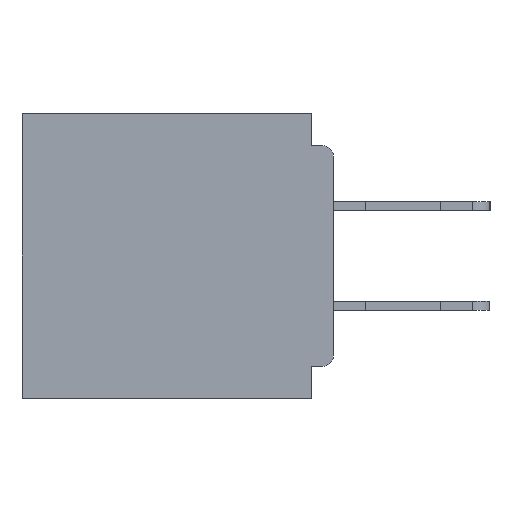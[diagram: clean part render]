
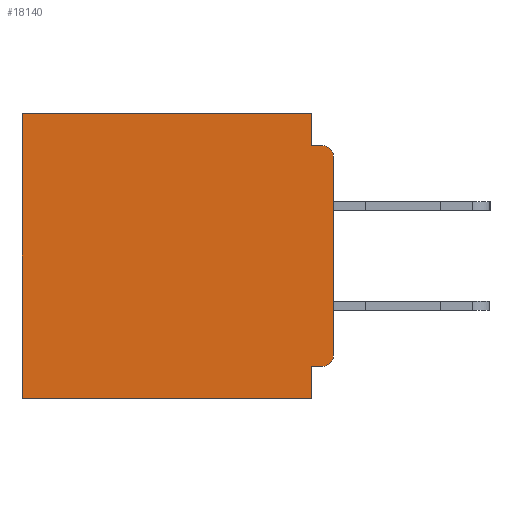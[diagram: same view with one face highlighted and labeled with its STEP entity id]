
A CAD part, left-side view. The second image highlights one B-rep face of the part: STEP entity #18140.
In plain terms, the highlighted planar face has unit normal (-1, 0, 0).
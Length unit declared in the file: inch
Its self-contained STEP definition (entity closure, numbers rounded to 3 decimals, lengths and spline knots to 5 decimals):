
#1460 = FACE_OUTER_BOUND ( 'NONE', #38488, .T. ) ;
#1604 = DIRECTION ( 'NONE',  ( 0., 0., -1. ) ) ;
#1790 = EDGE_CURVE ( 'NONE', #33776, #21565, #19119, .T. ) ;
#1946 = CARTESIAN_POINT ( 'NONE',  ( 0.3, 0., -0.4 ) ) ;
#2280 = LINE ( 'NONE', #10633, #11112 ) ;
#2460 = EDGE_CURVE ( 'NONE', #18944, #6877, #17499, .T. ) ;
#2597 = EDGE_CURVE ( 'NONE', #33776, #18944, #38839, .T. ) ;
#2975 = LINE ( 'NONE', #30619, #36220 ) ;
#3248 = CARTESIAN_POINT ( 'NONE',  ( 0.3, 0.015, -0.06 ) ) ;
#3604 = LINE ( 'NONE', #35738, #29031 ) ;
#5275 = VERTEX_POINT ( 'NONE', #12614 ) ;
#5469 = EDGE_CURVE ( 'NONE', #5275, #33750, #2280, .T. ) ;
#6628 = DIRECTION ( 'NONE',  ( 0., 0., -1. ) ) ;
#6877 = VERTEX_POINT ( 'NONE', #37821 ) ;
#7476 = DIRECTION ( 'NONE',  ( 0., 0., -1. ) ) ;
#7582 = PLANE ( 'NONE',  #20392 ) ;
#7740 = AXIS2_PLACEMENT_3D ( 'NONE', #25195, #25282, #26534 ) ;
#8827 = CARTESIAN_POINT ( 'NONE',  ( 0.3, 0.031, -0.355 ) ) ;
#10633 = CARTESIAN_POINT ( 'NONE',  ( 0.3, 0.437, -0.4 ) ) ;
#10864 = DIRECTION ( 'NONE',  ( 0., 0., -1. ) ) ;
#11112 = VECTOR ( 'NONE', #1604, 39.37008 ) ;
#12614 = CARTESIAN_POINT ( 'NONE',  ( 0.3, 0.437, 0. ) ) ;
#14399 = LINE ( 'NONE', #31849, #31014 ) ;
#14525 = CARTESIAN_POINT ( 'NONE',  ( 0.3, 0.031, 0. ) ) ;
#14537 = VERTEX_POINT ( 'NONE', #35769 ) ;
#16819 = ORIENTED_EDGE ( 'NONE', *, *, #2597, .F. ) ;
#17352 = VERTEX_POINT ( 'NONE', #14525 ) ;
#17499 = LINE ( 'NONE', #31809, #36252 ) ;
#17772 = LINE ( 'NONE', #1946, #41174 ) ;
#18140 = ADVANCED_FACE ( 'NONE', ( #1460 ), #7582, .F. ) ;
#18143 = VECTOR ( 'NONE', #19494, 39.37008 ) ;
#18463 = EDGE_CURVE ( 'NONE', #38807, #14537, #14399, .T. ) ;
#18944 = VERTEX_POINT ( 'NONE', #8827 ) ;
#18976 = CARTESIAN_POINT ( 'NONE',  ( 0.3, 0.031, -0.045 ) ) ;
#19119 = CIRCLE ( 'NONE', #7740, 0.015 ) ;
#19195 = LINE ( 'NONE', #42731, #18143 ) ;
#19494 = DIRECTION ( 'NONE',  ( 0., 1., 0. ) ) ;
#20392 = AXIS2_PLACEMENT_3D ( 'NONE', #20689, #30729, #10864 ) ;
#20689 = CARTESIAN_POINT ( 'NONE',  ( 0.3, 0., -0.4 ) ) ;
#20958 = CARTESIAN_POINT ( 'NONE',  ( 0.3, 0., -0.06 ) ) ;
#20993 = ORIENTED_EDGE ( 'NONE', *, *, #29904, .F. ) ;
#21375 = DIRECTION ( 'NONE',  ( 0., 1., 0. ) ) ;
#21565 = VERTEX_POINT ( 'NONE', #23058 ) ;
#21890 = CARTESIAN_POINT ( 'NONE',  ( 0.3, 0.015, -0.355 ) ) ;
#22543 = ORIENTED_EDGE ( 'NONE', *, *, #1790, .T. ) ;
#22721 = DIRECTION ( 'NONE',  ( 0., 0., -1. ) ) ;
#23058 = CARTESIAN_POINT ( 'NONE',  ( 0.3, 0., -0.34 ) ) ;
#23232 = EDGE_CURVE ( 'NONE', #17352, #5275, #3604, .T. ) ;
#23629 = ORIENTED_EDGE ( 'NONE', *, *, #33140, .F. ) ;
#24172 = AXIS2_PLACEMENT_3D ( 'NONE', #3248, #26444, #6628 ) ;
#25156 = ORIENTED_EDGE ( 'NONE', *, *, #18463, .F. ) ;
#25195 = CARTESIAN_POINT ( 'NONE',  ( 0.3, 0.015, -0.34 ) ) ;
#25282 = DIRECTION ( 'NONE',  ( -1., 0., 0. ) ) ;
#25742 = ORIENTED_EDGE ( 'NONE', *, *, #34652, .F. ) ;
#25830 = DIRECTION ( 'NONE',  ( 0., 1., 0. ) ) ;
#26357 = CIRCLE ( 'NONE', #24172, 0.015 ) ;
#26444 = DIRECTION ( 'NONE',  ( -1., 0., 0. ) ) ;
#26534 = DIRECTION ( 'NONE',  ( 0., 0., -1. ) ) ;
#27410 = VERTEX_POINT ( 'NONE', #20958 ) ;
#27508 = CARTESIAN_POINT ( 'NONE',  ( 0.3, 0., -0.355 ) ) ;
#28275 = CARTESIAN_POINT ( 'NONE',  ( 0.3, 0.437, -0.4 ) ) ;
#28468 = DIRECTION ( 'NONE',  ( 0., 0., -1. ) ) ;
#28781 = ORIENTED_EDGE ( 'NONE', *, *, #2460, .F. ) ;
#29031 = VECTOR ( 'NONE', #25830, 39.37008 ) ;
#29904 = EDGE_CURVE ( 'NONE', #17352, #38807, #2975, .T. ) ;
#29963 = VECTOR ( 'NONE', #21375, 39.37008 ) ;
#30619 = CARTESIAN_POINT ( 'NONE',  ( 0.3, 0.031, 0. ) ) ;
#30729 = DIRECTION ( 'NONE',  ( 1., 0., 0. ) ) ;
#31014 = VECTOR ( 'NONE', #42750, 39.37008 ) ;
#31444 = ORIENTED_EDGE ( 'NONE', *, *, #5469, .T. ) ;
#31809 = CARTESIAN_POINT ( 'NONE',  ( 0.3, 0.031, -0.4 ) ) ;
#31849 = CARTESIAN_POINT ( 'NONE',  ( 0.3, 0., -0.045 ) ) ;
#33140 = EDGE_CURVE ( 'NONE', #27410, #21565, #17772, .T. ) ;
#33750 = VERTEX_POINT ( 'NONE', #28275 ) ;
#33776 = VERTEX_POINT ( 'NONE', #21890 ) ;
#34652 = EDGE_CURVE ( 'NONE', #6877, #33750, #19195, .T. ) ;
#35738 = CARTESIAN_POINT ( 'NONE',  ( 0.3, 0., 0. ) ) ;
#35769 = CARTESIAN_POINT ( 'NONE',  ( 0.3, 0.015, -0.045 ) ) ;
#36220 = VECTOR ( 'NONE', #7476, 39.37008 ) ;
#36252 = VECTOR ( 'NONE', #22721, 39.37008 ) ;
#37821 = CARTESIAN_POINT ( 'NONE',  ( 0.3, 0.031, -0.4 ) ) ;
#38334 = EDGE_CURVE ( 'NONE', #27410, #14537, #26357, .T. ) ;
#38488 = EDGE_LOOP ( 'NONE', ( #23629, #40273, #25156, #20993, #40834, #31444, #25742, #28781, #16819, #22543 ) ) ;
#38807 = VERTEX_POINT ( 'NONE', #18976 ) ;
#38839 = LINE ( 'NONE', #27508, #29963 ) ;
#40273 = ORIENTED_EDGE ( 'NONE', *, *, #38334, .T. ) ;
#40834 = ORIENTED_EDGE ( 'NONE', *, *, #23232, .T. ) ;
#41174 = VECTOR ( 'NONE', #28468, 39.37008 ) ;
#42731 = CARTESIAN_POINT ( 'NONE',  ( 0.3, 0., -0.4 ) ) ;
#42750 = DIRECTION ( 'NONE',  ( 0., -1., 0. ) ) ;
